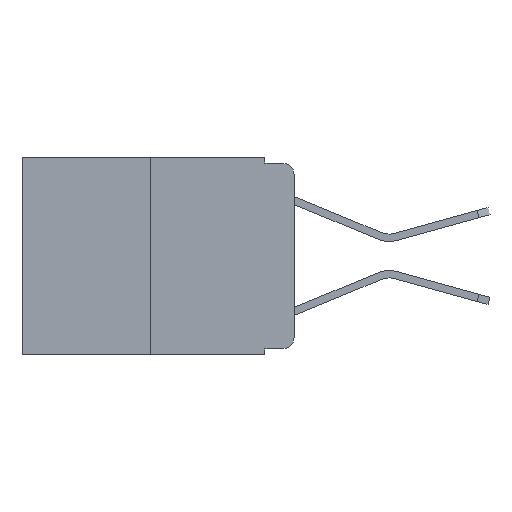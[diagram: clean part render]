
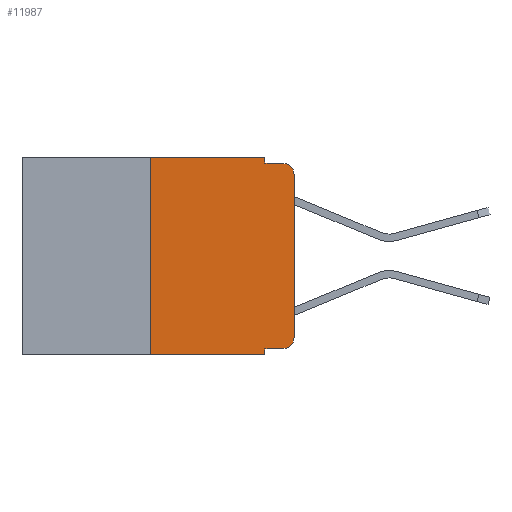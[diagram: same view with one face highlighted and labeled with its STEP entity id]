
A CAD part, left-side view. The second image highlights one B-rep face of the part: STEP entity #11987.
In plain terms, the highlighted planar face has unit normal (-1, 0, 0).
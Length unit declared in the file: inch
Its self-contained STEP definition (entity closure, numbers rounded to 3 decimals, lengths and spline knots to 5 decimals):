
#106 = VECTOR ( 'NONE', #7930, 39.37008 ) ;
#431 = VECTOR ( 'NONE', #8675, 39.37008 ) ;
#499 = CARTESIAN_POINT ( 'NONE',  ( 0., 0.051, -0.01 ) ) ;
#588 = DIRECTION ( 'NONE',  ( 0., -1., 0. ) ) ;
#767 = CARTESIAN_POINT ( 'NONE',  ( 0., 0.051, -0.01 ) ) ;
#890 = VECTOR ( 'NONE', #7318, 39.37008 ) ;
#932 = VERTEX_POINT ( 'NONE', #2113 ) ;
#1019 = ORIENTED_EDGE ( 'NONE', *, *, #10240, .F. ) ;
#1073 = LINE ( 'NONE', #499, #4263 ) ;
#1111 = ORIENTED_EDGE ( 'NONE', *, *, #9935, .T. ) ;
#1710 = ORIENTED_EDGE ( 'NONE', *, *, #10235, .F. ) ;
#1821 = DIRECTION ( 'NONE',  ( 0., -1., 0. ) ) ;
#2113 = CARTESIAN_POINT ( 'NONE',  ( 0., 0., -0.313 ) ) ;
#2200 = CARTESIAN_POINT ( 'NONE',  ( 0., 0.051, -0.333 ) ) ;
#2790 = ORIENTED_EDGE ( 'NONE', *, *, #10211, .T. ) ;
#2835 = CARTESIAN_POINT ( 'NONE',  ( 0., 0.02, -0.01 ) ) ;
#2863 = CARTESIAN_POINT ( 'NONE',  ( 0., 0.051, 0. ) ) ;
#3187 = ORIENTED_EDGE ( 'NONE', *, *, #9658, .F. ) ;
#3406 = CARTESIAN_POINT ( 'NONE',  ( 0., 0.051, -0.333 ) ) ;
#3465 = VERTEX_POINT ( 'NONE', #14366 ) ;
#4263 = VECTOR ( 'NONE', #588, 39.37008 ) ;
#4661 = ORIENTED_EDGE ( 'NONE', *, *, #10218, .F. ) ;
#4666 = VECTOR ( 'NONE', #13701, 39.37008 ) ;
#4681 = CARTESIAN_POINT ( 'NONE',  ( 0., 0.051, 0. ) ) ;
#4741 = DIRECTION ( 'NONE',  ( -1., 0., 0. ) ) ;
#5467 = VERTEX_POINT ( 'NONE', #2863 ) ;
#5642 = VECTOR ( 'NONE', #1821, 39.37008 ) ;
#5962 = VERTEX_POINT ( 'NONE', #10454 ) ;
#6002 = VERTEX_POINT ( 'NONE', #2835 ) ;
#6028 = CARTESIAN_POINT ( 'NONE',  ( 0., 0.051, 0. ) ) ;
#6066 = LINE ( 'NONE', #14778, #5642 ) ;
#6598 = CARTESIAN_POINT ( 'NONE',  ( 0., 0.473, -0.343 ) ) ;
#7318 = DIRECTION ( 'NONE',  ( 0., 0., 1. ) ) ;
#7429 = DIRECTION ( 'NONE',  ( -1., 0., 0. ) ) ;
#7454 = CARTESIAN_POINT ( 'NONE',  ( 0., 0.02, -0.333 ) ) ;
#7474 = ORIENTED_EDGE ( 'NONE', *, *, #10261, .F. ) ;
#7478 = DIRECTION ( 'NONE',  ( 1., 0., 0. ) ) ;
#7722 = LINE ( 'NONE', #3406, #431 ) ;
#7875 = EDGE_LOOP ( 'NONE', ( #9169, #2790, #4661, #1710, #3187, #1019, #1111, #7474, #11940, #14911 ) ) ;
#7930 = DIRECTION ( 'NONE',  ( 0., -1., 0. ) ) ;
#7993 = VERTEX_POINT ( 'NONE', #15121 ) ;
#8545 = CARTESIAN_POINT ( 'NONE',  ( 0., 0.051, -0.343 ) ) ;
#8675 = DIRECTION ( 'NONE',  ( 0., -1., 0. ) ) ;
#9169 = ORIENTED_EDGE ( 'NONE', *, *, #10189, .T. ) ;
#9259 = AXIS2_PLACEMENT_3D ( 'NONE', #12490, #4741, #13760 ) ;
#9658 = EDGE_CURVE ( 'NONE', #5962, #5467, #6066, .T. ) ;
#9935 = EDGE_CURVE ( 'NONE', #3465, #13665, #10697, .T. ) ;
#10045 = CARTESIAN_POINT ( 'NONE',  ( 0., 0.473, 0. ) ) ;
#10189 = EDGE_CURVE ( 'NONE', #932, #7993, #11589, .T. ) ;
#10211 = EDGE_CURVE ( 'NONE', #7993, #6002, #14543, .T. ) ;
#10218 = EDGE_CURVE ( 'NONE', #11992, #6002, #1073, .T. ) ;
#10235 = EDGE_CURVE ( 'NONE', #5467, #11992, #14370, .T. ) ;
#10240 = EDGE_CURVE ( 'NONE', #3465, #5962, #14936, .T. ) ;
#10261 = EDGE_CURVE ( 'NONE', #16525, #13665, #13978, .T. ) ;
#10263 = EDGE_CURVE ( 'NONE', #16525, #12463, #7722, .T. ) ;
#10272 = EDGE_CURVE ( 'NONE', #12463, #932, #13562, .T. ) ;
#10454 = CARTESIAN_POINT ( 'NONE',  ( 0., 0.25, 0. ) ) ;
#10602 = VECTOR ( 'NONE', #15031, 39.37008 ) ;
#10697 = LINE ( 'NONE', #6598, #106 ) ;
#10715 = FACE_OUTER_BOUND ( 'NONE', #7875, .T. ) ;
#11002 = VECTOR ( 'NONE', #14980, 39.37008 ) ;
#11589 = LINE ( 'NONE', #12431, #4666 ) ;
#11940 = ORIENTED_EDGE ( 'NONE', *, *, #10263, .T. ) ;
#11987 = ADVANCED_FACE ( 'NONE', ( #10715 ), #12603, .F. ) ;
#11992 = VERTEX_POINT ( 'NONE', #767 ) ;
#12431 = CARTESIAN_POINT ( 'NONE',  ( 0., 0., 0. ) ) ;
#12463 = VERTEX_POINT ( 'NONE', #7454 ) ;
#12490 = CARTESIAN_POINT ( 'NONE',  ( 0., 0.02, -0.03 ) ) ;
#12603 = PLANE ( 'NONE',  #15872 ) ;
#13517 = AXIS2_PLACEMENT_3D ( 'NONE', #15088, #7429, #16345 ) ;
#13562 = CIRCLE ( 'NONE', #13517, 0.02 ) ;
#13665 = VERTEX_POINT ( 'NONE', #8545 ) ;
#13701 = DIRECTION ( 'NONE',  ( 0., 0., 1. ) ) ;
#13703 = CARTESIAN_POINT ( 'NONE',  ( 0., 0.25, 0. ) ) ;
#13760 = DIRECTION ( 'NONE',  ( 0., 0., -1. ) ) ;
#13978 = LINE ( 'NONE', #6028, #10602 ) ;
#14366 = CARTESIAN_POINT ( 'NONE',  ( 0., 0.25, -0.343 ) ) ;
#14370 = LINE ( 'NONE', #4681, #11002 ) ;
#14543 = CIRCLE ( 'NONE', #9259, 0.02 ) ;
#14778 = CARTESIAN_POINT ( 'NONE',  ( 0., 0.473, 0. ) ) ;
#14911 = ORIENTED_EDGE ( 'NONE', *, *, #10272, .T. ) ;
#14936 = LINE ( 'NONE', #13703, #890 ) ;
#14980 = DIRECTION ( 'NONE',  ( 0., 0., -1. ) ) ;
#15031 = DIRECTION ( 'NONE',  ( 0., 0., -1. ) ) ;
#15088 = CARTESIAN_POINT ( 'NONE',  ( 0., 0.02, -0.313 ) ) ;
#15121 = CARTESIAN_POINT ( 'NONE',  ( 0., 0., -0.03 ) ) ;
#15872 = AXIS2_PLACEMENT_3D ( 'NONE', #10045, #7478, #16386 ) ;
#16345 = DIRECTION ( 'NONE',  ( 0., 0., -1. ) ) ;
#16386 = DIRECTION ( 'NONE',  ( 0., 0., -1. ) ) ;
#16525 = VERTEX_POINT ( 'NONE', #2200 ) ;
